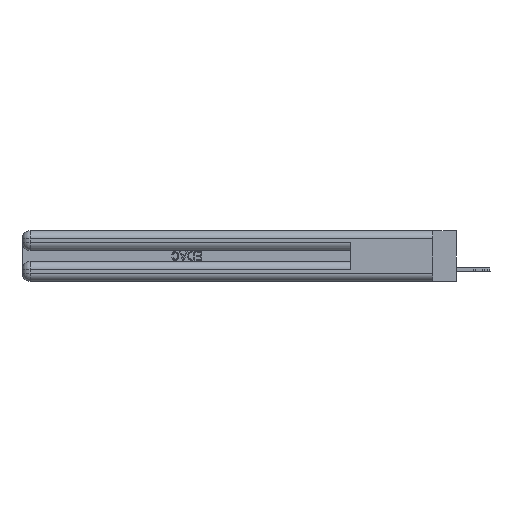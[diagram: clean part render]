
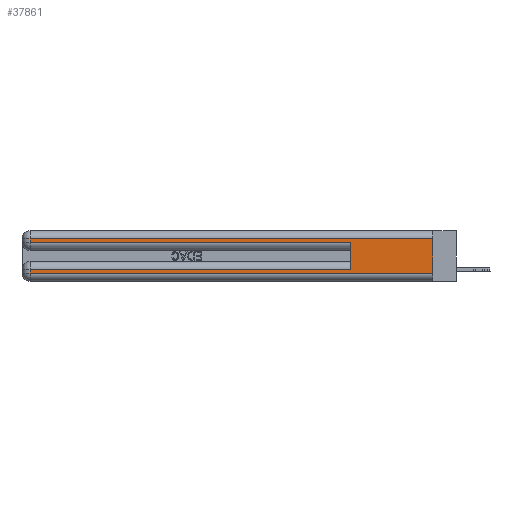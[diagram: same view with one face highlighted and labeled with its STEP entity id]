
A CAD part, left-side view. The second image highlights one B-rep face of the part: STEP entity #37861.
In plain terms, the highlighted planar face has unit normal (-1, 0, 0).
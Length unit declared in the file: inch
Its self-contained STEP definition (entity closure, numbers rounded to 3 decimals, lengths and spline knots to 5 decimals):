
#82 = ORIENTED_EDGE ( 'NONE', *, *, #16146, .T. ) ;
#557 = CARTESIAN_POINT ( 'NONE',  ( 0., 0.6, 0.285 ) ) ;
#681 = LINE ( 'NONE', #14076, #25444 ) ;
#687 = VERTEX_POINT ( 'NONE', #32258 ) ;
#806 = CARTESIAN_POINT ( 'NONE',  ( 0., 0., 0.06 ) ) ;
#2245 = LINE ( 'NONE', #33179, #40066 ) ;
#2629 = DIRECTION ( 'NONE',  ( 0., 0., 1. ) ) ;
#3093 = CARTESIAN_POINT ( 'NONE',  ( 0., 2.94, 0.37 ) ) ;
#3329 = LINE ( 'NONE', #13596, #36639 ) ;
#4001 = CARTESIAN_POINT ( 'NONE',  ( 0., 0., 0.37 ) ) ;
#4340 = FACE_OUTER_BOUND ( 'NONE', #20606, .T. ) ;
#6498 = VERTEX_POINT ( 'NONE', #557 ) ;
#7021 = VECTOR ( 'NONE', #38376, 39.37008 ) ;
#7371 = PLANE ( 'NONE',  #33388 ) ;
#7856 = EDGE_CURVE ( 'NONE', #33790, #39876, #13388, .T. ) ;
#9393 = CARTESIAN_POINT ( 'NONE',  ( 0., 2.94, 0.085 ) ) ;
#9562 = CARTESIAN_POINT ( 'NONE',  ( 0., 0., 0.37 ) ) ;
#10476 = DIRECTION ( 'NONE',  ( 0., 0., -1. ) ) ;
#11600 = VERTEX_POINT ( 'NONE', #806 ) ;
#11960 = ORIENTED_EDGE ( 'NONE', *, *, #7856, .T. ) ;
#12735 = CARTESIAN_POINT ( 'NONE',  ( 0., 0.6, 0.085 ) ) ;
#13359 = CARTESIAN_POINT ( 'NONE',  ( 0., 0., 0.285 ) ) ;
#13388 = LINE ( 'NONE', #15218, #27586 ) ;
#13596 = CARTESIAN_POINT ( 'NONE',  ( 0., 0., 0.06 ) ) ;
#13847 = DIRECTION ( 'NONE',  ( 1., 0., 0. ) ) ;
#14076 = CARTESIAN_POINT ( 'NONE',  ( 0., 2.94, 0.37 ) ) ;
#14878 = VECTOR ( 'NONE', #32846, 39.37008 ) ;
#15218 = CARTESIAN_POINT ( 'NONE',  ( 0., 0., 0.31 ) ) ;
#15473 = ORIENTED_EDGE ( 'NONE', *, *, #32283, .F. ) ;
#16146 = EDGE_CURVE ( 'NONE', #37969, #11600, #3329, .T. ) ;
#16585 = EDGE_CURVE ( 'NONE', #687, #6498, #18407, .T. ) ;
#16806 = CARTESIAN_POINT ( 'NONE',  ( 0., 0., 0.31 ) ) ;
#16871 = DIRECTION ( 'NONE',  ( 0., 1., 0. ) ) ;
#17778 = ORIENTED_EDGE ( 'NONE', *, *, #23776, .T. ) ;
#18200 = VERTEX_POINT ( 'NONE', #9393 ) ;
#18407 = LINE ( 'NONE', #13359, #14878 ) ;
#19431 = EDGE_CURVE ( 'NONE', #18200, #37969, #24683, .T. ) ;
#20606 = EDGE_LOOP ( 'NONE', ( #25725, #11960, #17778, #39039, #15473, #20674, #26197, #82 ) ) ;
#20674 = ORIENTED_EDGE ( 'NONE', *, *, #39000, .T. ) ;
#21073 = DIRECTION ( 'NONE',  ( 0., -1., 0. ) ) ;
#22864 = EDGE_CURVE ( 'NONE', #33790, #11600, #24999, .T. ) ;
#23776 = EDGE_CURVE ( 'NONE', #39876, #687, #681, .T. ) ;
#23868 = DIRECTION ( 'NONE',  ( 0., 1., 0. ) ) ;
#24683 = LINE ( 'NONE', #3093, #7021 ) ;
#24999 = LINE ( 'NONE', #9562, #25523 ) ;
#25444 = VECTOR ( 'NONE', #26928, 39.37008 ) ;
#25523 = VECTOR ( 'NONE', #33367, 39.37008 ) ;
#25725 = ORIENTED_EDGE ( 'NONE', *, *, #22864, .F. ) ;
#26197 = ORIENTED_EDGE ( 'NONE', *, *, #19431, .T. ) ;
#26928 = DIRECTION ( 'NONE',  ( 0., 0., -1. ) ) ;
#26962 = LINE ( 'NONE', #37763, #33551 ) ;
#27586 = VECTOR ( 'NONE', #23868, 39.37008 ) ;
#32258 = CARTESIAN_POINT ( 'NONE',  ( 0., 2.94, 0.285 ) ) ;
#32283 = EDGE_CURVE ( 'NONE', #41410, #6498, #26962, .T. ) ;
#32846 = DIRECTION ( 'NONE',  ( 0., -1., 0. ) ) ;
#33179 = CARTESIAN_POINT ( 'NONE',  ( 0., 0., 0.085 ) ) ;
#33367 = DIRECTION ( 'NONE',  ( 0., 0., -1. ) ) ;
#33388 = AXIS2_PLACEMENT_3D ( 'NONE', #4001, #13847, #10476 ) ;
#33492 = CARTESIAN_POINT ( 'NONE',  ( 0., 2.94, 0.06 ) ) ;
#33551 = VECTOR ( 'NONE', #2629, 39.37008 ) ;
#33790 = VERTEX_POINT ( 'NONE', #16806 ) ;
#36639 = VECTOR ( 'NONE', #21073, 39.37008 ) ;
#37763 = CARTESIAN_POINT ( 'NONE',  ( 0., 0.6, 0.145 ) ) ;
#37861 = ADVANCED_FACE ( 'NONE', ( #4340 ), #7371, .F. ) ;
#37969 = VERTEX_POINT ( 'NONE', #33492 ) ;
#38376 = DIRECTION ( 'NONE',  ( 0., 0., -1. ) ) ;
#39000 = EDGE_CURVE ( 'NONE', #41410, #18200, #2245, .T. ) ;
#39039 = ORIENTED_EDGE ( 'NONE', *, *, #16585, .T. ) ;
#39876 = VERTEX_POINT ( 'NONE', #40655 ) ;
#40066 = VECTOR ( 'NONE', #16871, 39.37008 ) ;
#40655 = CARTESIAN_POINT ( 'NONE',  ( 0., 2.94, 0.31 ) ) ;
#41410 = VERTEX_POINT ( 'NONE', #12735 ) ;
